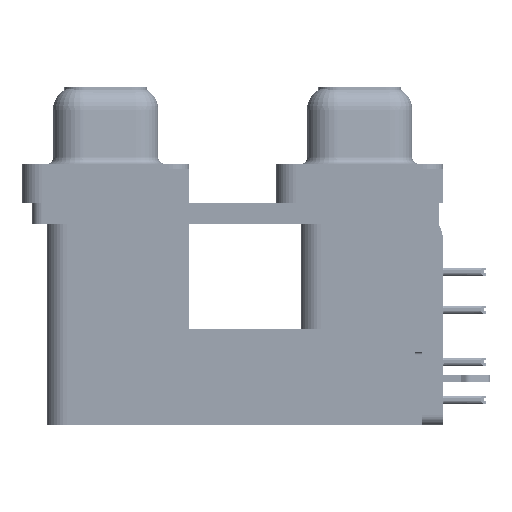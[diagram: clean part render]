
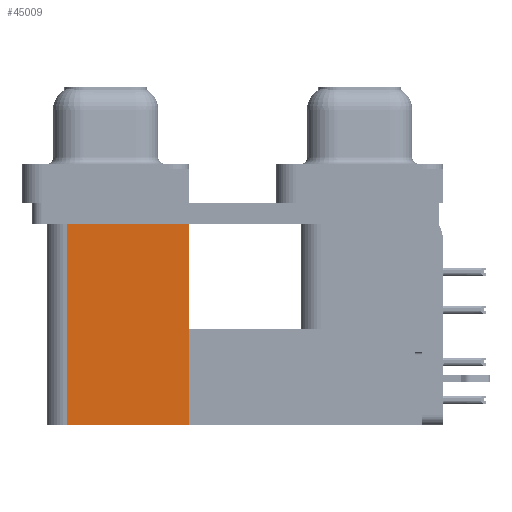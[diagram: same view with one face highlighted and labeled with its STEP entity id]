
A CAD part, left-side view. The second image highlights one B-rep face of the part: STEP entity #45009.
In plain terms, the highlighted planar face has unit normal (-1, 0, 0).
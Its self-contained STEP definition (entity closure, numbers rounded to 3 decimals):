
#4594 = PLANE ( 'NONE',  #16234 ) ;
#5866 = VERTEX_POINT ( 'NONE', #54648 ) ;
#8237 = LINE ( 'NONE', #60042, #16170 ) ;
#11016 = VECTOR ( 'NONE', #58016, 1000. ) ;
#11242 = CARTESIAN_POINT ( 'NONE',  ( 3.79, 12.775, -2.5 ) ) ;
#11548 = CARTESIAN_POINT ( 'NONE',  ( 3.79, 12.775, -19.2 ) ) ;
#14520 = ORIENTED_EDGE ( 'NONE', *, *, #44392, .F. ) ;
#16170 = VECTOR ( 'NONE', #18687, 1000. ) ;
#16234 = AXIS2_PLACEMENT_3D ( 'NONE', #11548, #51756, #28180 ) ;
#16295 = LINE ( 'NONE', #11242, #11016 ) ;
#18481 = EDGE_LOOP ( 'NONE', ( #22802, #14520, #18518, #68602 ) ) ;
#18518 = ORIENTED_EDGE ( 'NONE', *, *, #44914, .F. ) ;
#18687 = DIRECTION ( 'NONE',  ( 0., 0., 1. ) ) ;
#21271 = DIRECTION ( 'NONE',  ( 0., 1., 0. ) ) ;
#22802 = ORIENTED_EDGE ( 'NONE', *, *, #72583, .T. ) ;
#26422 = VECTOR ( 'NONE', #57855, 1000. ) ;
#28180 = DIRECTION ( 'NONE',  ( 0., 0., -1. ) ) ;
#28486 = LINE ( 'NONE', #58626, #26422 ) ;
#36794 = VERTEX_POINT ( 'NONE', #52594 ) ;
#38418 = VECTOR ( 'NONE', #21271, 1000. ) ;
#38587 = VERTEX_POINT ( 'NONE', #48259 ) ;
#44392 = EDGE_CURVE ( 'NONE', #38587, #5866, #8237, .T. ) ;
#44914 = EDGE_CURVE ( 'NONE', #49888, #38587, #50229, .T. ) ;
#45009 = ADVANCED_FACE ( 'NONE', ( #52893 ), #4594, .F. ) ;
#48259 = CARTESIAN_POINT ( 'NONE',  ( 3.79, 21.975, -19.2 ) ) ;
#48819 = EDGE_CURVE ( 'NONE', #49888, #36794, #28486, .T. ) ;
#49888 = VERTEX_POINT ( 'NONE', #70609 ) ;
#50229 = LINE ( 'NONE', #74176, #38418 ) ;
#51756 = DIRECTION ( 'NONE',  ( 1., 0., 0. ) ) ;
#52594 = CARTESIAN_POINT ( 'NONE',  ( 3.79, 12.775, -2.5 ) ) ;
#52893 = FACE_OUTER_BOUND ( 'NONE', #18481, .T. ) ;
#54648 = CARTESIAN_POINT ( 'NONE',  ( 3.79, 21.975, -2.5 ) ) ;
#57855 = DIRECTION ( 'NONE',  ( 0., 0., 1. ) ) ;
#58016 = DIRECTION ( 'NONE',  ( 0., 1., 0. ) ) ;
#58626 = CARTESIAN_POINT ( 'NONE',  ( 3.79, 12.775, -19.2 ) ) ;
#60042 = CARTESIAN_POINT ( 'NONE',  ( 3.79, 21.975, -19.2 ) ) ;
#68602 = ORIENTED_EDGE ( 'NONE', *, *, #48819, .T. ) ;
#70609 = CARTESIAN_POINT ( 'NONE',  ( 3.79, 12.775, -19.2 ) ) ;
#72583 = EDGE_CURVE ( 'NONE', #36794, #5866, #16295, .T. ) ;
#74176 = CARTESIAN_POINT ( 'NONE',  ( 3.79, 12.775, -19.2 ) ) ;
